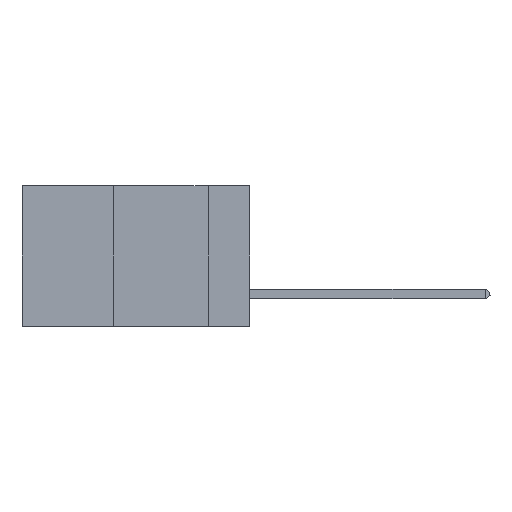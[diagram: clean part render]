
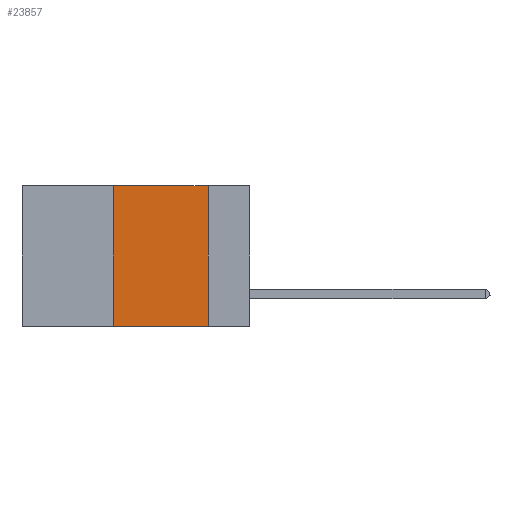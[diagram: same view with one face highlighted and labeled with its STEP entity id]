
A CAD part, left-side view. The second image highlights one B-rep face of the part: STEP entity #23857.
In plain terms, the highlighted planar face has unit normal (-1, 0, 0).
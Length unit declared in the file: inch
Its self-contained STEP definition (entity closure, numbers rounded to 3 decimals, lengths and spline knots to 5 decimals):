
#129 = VERTEX_POINT ( 'NONE', #20503 ) ;
#641 = CARTESIAN_POINT ( 'NONE',  ( 0., 0.6, 0. ) ) ;
#726 = DIRECTION ( 'NONE',  ( 0., 0., -1. ) ) ;
#1045 = AXIS2_PLACEMENT_3D ( 'NONE', #641, #18518, #726 ) ;
#1574 = VECTOR ( 'NONE', #2078, 39.37008 ) ;
#1725 = EDGE_LOOP ( 'NONE', ( #9265, #2102, #7226, #11044 ) ) ;
#2078 = DIRECTION ( 'NONE',  ( 0., 0., 1. ) ) ;
#2102 = ORIENTED_EDGE ( 'NONE', *, *, #11577, .F. ) ;
#2277 = VECTOR ( 'NONE', #16802, 39.37008 ) ;
#4209 = CARTESIAN_POINT ( 'NONE',  ( 0., 0.36, 0. ) ) ;
#5041 = VERTEX_POINT ( 'NONE', #20549 ) ;
#6440 = VECTOR ( 'NONE', #17881, 39.37008 ) ;
#7226 = ORIENTED_EDGE ( 'NONE', *, *, #14604, .F. ) ;
#9265 = ORIENTED_EDGE ( 'NONE', *, *, #21126, .F. ) ;
#9475 = CARTESIAN_POINT ( 'NONE',  ( 0., 0.6, -0.37 ) ) ;
#10521 = EDGE_CURVE ( 'NONE', #5041, #129, #15027, .T. ) ;
#10777 = VERTEX_POINT ( 'NONE', #23498 ) ;
#11044 = ORIENTED_EDGE ( 'NONE', *, *, #10521, .T. ) ;
#11577 = EDGE_CURVE ( 'NONE', #23076, #10777, #22353, .T. ) ;
#13926 = CARTESIAN_POINT ( 'NONE',  ( 0., 0.36, 0. ) ) ;
#14604 = EDGE_CURVE ( 'NONE', #5041, #23076, #16423, .T. ) ;
#14735 = CARTESIAN_POINT ( 'NONE',  ( 0., 0.6, 0. ) ) ;
#15027 = LINE ( 'NONE', #9475, #21825 ) ;
#16324 = LINE ( 'NONE', #20032, #6440 ) ;
#16423 = LINE ( 'NONE', #13926, #1574 ) ;
#16802 = DIRECTION ( 'NONE',  ( 0., -1., 0. ) ) ;
#17701 = FACE_OUTER_BOUND ( 'NONE', #1725, .T. ) ;
#17881 = DIRECTION ( 'NONE',  ( 0., 0., -1. ) ) ;
#18518 = DIRECTION ( 'NONE',  ( 1., 0., 0. ) ) ;
#20032 = CARTESIAN_POINT ( 'NONE',  ( 0., 0.11, 0. ) ) ;
#20496 = PLANE ( 'NONE',  #1045 ) ;
#20503 = CARTESIAN_POINT ( 'NONE',  ( 0., 0.11, -0.37 ) ) ;
#20549 = CARTESIAN_POINT ( 'NONE',  ( 0., 0.36, -0.37 ) ) ;
#21126 = EDGE_CURVE ( 'NONE', #10777, #129, #16324, .T. ) ;
#21825 = VECTOR ( 'NONE', #23254, 39.37008 ) ;
#22353 = LINE ( 'NONE', #14735, #2277 ) ;
#23076 = VERTEX_POINT ( 'NONE', #4209 ) ;
#23254 = DIRECTION ( 'NONE',  ( 0., -1., 0. ) ) ;
#23498 = CARTESIAN_POINT ( 'NONE',  ( 0., 0.11, 0. ) ) ;
#23857 = ADVANCED_FACE ( 'NONE', ( #17701 ), #20496, .F. ) ;
